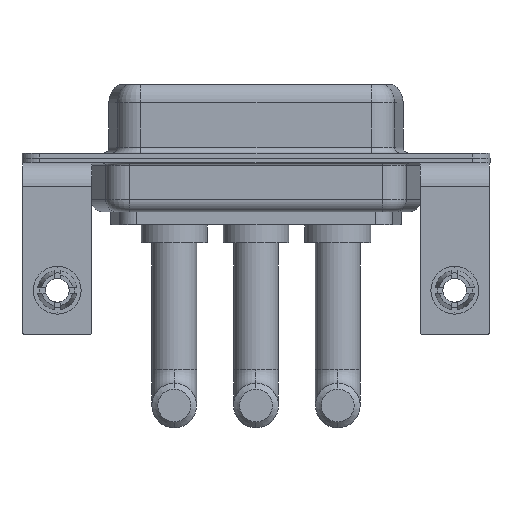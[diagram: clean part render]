
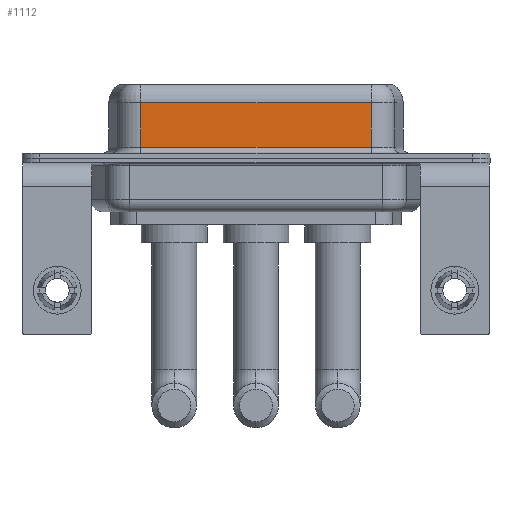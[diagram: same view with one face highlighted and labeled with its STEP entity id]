
A CAD part, front view. The second image highlights one B-rep face of the part: STEP entity #1112.
In plain terms, the highlighted planar face has unit normal (0, -1, 0).
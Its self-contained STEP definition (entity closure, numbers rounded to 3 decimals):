
#70 = PLANE ( 'NONE',  #12106 ) ;
#189 = CARTESIAN_POINT ( 'NONE',  ( 26.287, -3.95, 0.9 ) ) ;
#454 = VECTOR ( 'NONE', #6750, 1000. ) ;
#1112 = ADVANCED_FACE ( 'NONE', ( #10049 ), #70, .F. ) ;
#1441 = LINE ( 'NONE', #13814, #14068 ) ;
#1974 = DIRECTION ( 'NONE',  ( -1., 0., 0. ) ) ;
#2011 = EDGE_CURVE ( 'NONE', #10415, #9639, #13303, .T. ) ;
#2029 = EDGE_LOOP ( 'NONE', ( #12592, #12529, #7173, #8144 ) ) ;
#2217 = VERTEX_POINT ( 'NONE', #189 ) ;
#2471 = CARTESIAN_POINT ( 'NONE',  ( 26.287, -3.95, 4.65 ) ) ;
#3079 = VECTOR ( 'NONE', #8851, 1000. ) ;
#3118 = CARTESIAN_POINT ( 'NONE',  ( 26.287, -3.95, 6.4 ) ) ;
#4291 = LINE ( 'NONE', #14447, #3079 ) ;
#4386 = DIRECTION ( 'NONE',  ( 0., 0., 1. ) ) ;
#4551 = EDGE_CURVE ( 'NONE', #13322, #2217, #12349, .T. ) ;
#6750 = DIRECTION ( 'NONE',  ( 1., 0., 0. ) ) ;
#6821 = CARTESIAN_POINT ( 'NONE',  ( 26.287, -3.95, 0.9 ) ) ;
#7018 = DIRECTION ( 'NONE',  ( 0., 0., -1. ) ) ;
#7173 = ORIENTED_EDGE ( 'NONE', *, *, #9938, .T. ) ;
#8144 = ORIENTED_EDGE ( 'NONE', *, *, #4551, .T. ) ;
#8851 = DIRECTION ( 'NONE',  ( 0., 0., -1. ) ) ;
#9247 = CARTESIAN_POINT ( 'NONE',  ( 7.013, -3.95, 4.65 ) ) ;
#9639 = VERTEX_POINT ( 'NONE', #9247 ) ;
#9938 = EDGE_CURVE ( 'NONE', #9639, #13322, #4291, .T. ) ;
#10049 = FACE_OUTER_BOUND ( 'NONE', #2029, .T. ) ;
#10415 = VERTEX_POINT ( 'NONE', #2471 ) ;
#10465 = EDGE_CURVE ( 'NONE', #10415, #2217, #1441, .T. ) ;
#12106 = AXIS2_PLACEMENT_3D ( 'NONE', #3118, #14609, #4386 ) ;
#12173 = CARTESIAN_POINT ( 'NONE',  ( 26.287, -3.95, 4.65 ) ) ;
#12349 = LINE ( 'NONE', #6821, #454 ) ;
#12529 = ORIENTED_EDGE ( 'NONE', *, *, #2011, .T. ) ;
#12592 = ORIENTED_EDGE ( 'NONE', *, *, #10465, .F. ) ;
#12600 = VECTOR ( 'NONE', #1974, 1000. ) ;
#13303 = LINE ( 'NONE', #12173, #12600 ) ;
#13322 = VERTEX_POINT ( 'NONE', #14398 ) ;
#13814 = CARTESIAN_POINT ( 'NONE',  ( 26.287, -3.95, 6.4 ) ) ;
#14068 = VECTOR ( 'NONE', #7018, 1000. ) ;
#14398 = CARTESIAN_POINT ( 'NONE',  ( 7.013, -3.95, 0.9 ) ) ;
#14447 = CARTESIAN_POINT ( 'NONE',  ( 7.013, -3.95, 6.4 ) ) ;
#14609 = DIRECTION ( 'NONE',  ( 0., 1., 0. ) ) ;
